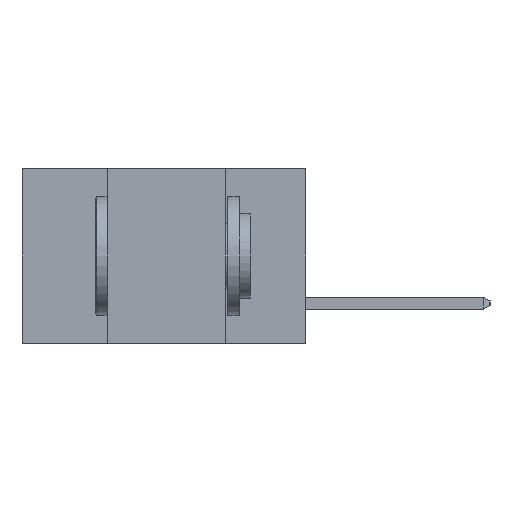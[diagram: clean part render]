
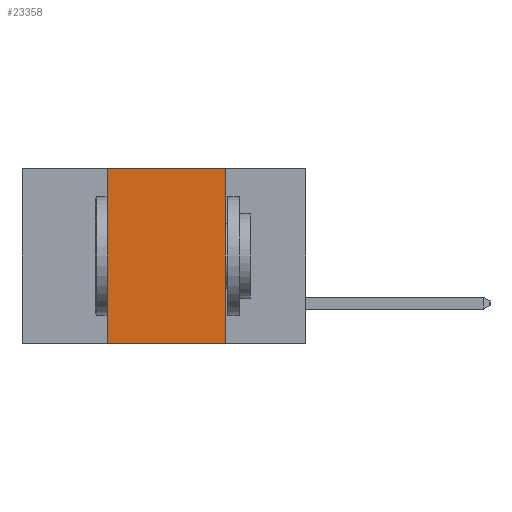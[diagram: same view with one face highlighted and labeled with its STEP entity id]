
A CAD part, left-side view. The second image highlights one B-rep face of the part: STEP entity #23358.
In plain terms, the highlighted planar face has unit normal (-1, 0, 0).
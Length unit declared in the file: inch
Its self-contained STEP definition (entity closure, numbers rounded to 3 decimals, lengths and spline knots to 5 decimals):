
#39 = DIRECTION ( 'NONE',  ( 0., 0., -1. ) ) ;
#115 = CARTESIAN_POINT ( 'NONE',  ( 0., 0.42, -0.37 ) ) ;
#291 = LINE ( 'NONE', #10099, #11325 ) ;
#905 = CARTESIAN_POINT ( 'NONE',  ( 0., 0.17, 0. ) ) ;
#2375 = EDGE_CURVE ( 'NONE', #19141, #6452, #291, .T. ) ;
#3187 = VERTEX_POINT ( 'NONE', #23948 ) ;
#4057 = EDGE_CURVE ( 'NONE', #3187, #21270, #27892, .T. ) ;
#4259 = DIRECTION ( 'NONE',  ( 0., 0., -1. ) ) ;
#4649 = VECTOR ( 'NONE', #28094, 39.37008 ) ;
#6452 = VERTEX_POINT ( 'NONE', #7608 ) ;
#7299 = LINE ( 'NONE', #24254, #13763 ) ;
#7608 = CARTESIAN_POINT ( 'NONE',  ( 0., 0.17, -0.37 ) ) ;
#7925 = ORIENTED_EDGE ( 'NONE', *, *, #4057, .F. ) ;
#9216 = ORIENTED_EDGE ( 'NONE', *, *, #2375, .T. ) ;
#10099 = CARTESIAN_POINT ( 'NONE',  ( 0., 0.6, -0.37 ) ) ;
#11325 = VECTOR ( 'NONE', #18725, 39.37008 ) ;
#11797 = EDGE_CURVE ( 'NONE', #21270, #6452, #7299, .T. ) ;
#11799 = AXIS2_PLACEMENT_3D ( 'NONE', #15202, #17380, #4259 ) ;
#12043 = LINE ( 'NONE', #22935, #17848 ) ;
#13763 = VECTOR ( 'NONE', #39, 39.37008 ) ;
#15202 = CARTESIAN_POINT ( 'NONE',  ( 0., 0.6, 0. ) ) ;
#17380 = DIRECTION ( 'NONE',  ( 1., 0., 0. ) ) ;
#17848 = VECTOR ( 'NONE', #22843, 39.37008 ) ;
#18725 = DIRECTION ( 'NONE',  ( 0., -1., 0. ) ) ;
#19141 = VERTEX_POINT ( 'NONE', #115 ) ;
#21070 = ORIENTED_EDGE ( 'NONE', *, *, #11797, .F. ) ;
#21270 = VERTEX_POINT ( 'NONE', #905 ) ;
#21791 = EDGE_LOOP ( 'NONE', ( #21070, #7925, #24651, #9216 ) ) ;
#22843 = DIRECTION ( 'NONE',  ( 0., 0., 1. ) ) ;
#22935 = CARTESIAN_POINT ( 'NONE',  ( 0., 0.42, 0. ) ) ;
#23358 = ADVANCED_FACE ( 'NONE', ( #27316 ), #28207, .F. ) ;
#23948 = CARTESIAN_POINT ( 'NONE',  ( 0., 0.42, 0. ) ) ;
#24254 = CARTESIAN_POINT ( 'NONE',  ( 0., 0.17, 0. ) ) ;
#24651 = ORIENTED_EDGE ( 'NONE', *, *, #27249, .F. ) ;
#27249 = EDGE_CURVE ( 'NONE', #19141, #3187, #12043, .T. ) ;
#27316 = FACE_OUTER_BOUND ( 'NONE', #21791, .T. ) ;
#27892 = LINE ( 'NONE', #28055, #4649 ) ;
#28055 = CARTESIAN_POINT ( 'NONE',  ( 0., 0.6, 0. ) ) ;
#28094 = DIRECTION ( 'NONE',  ( 0., -1., 0. ) ) ;
#28207 = PLANE ( 'NONE',  #11799 ) ;
